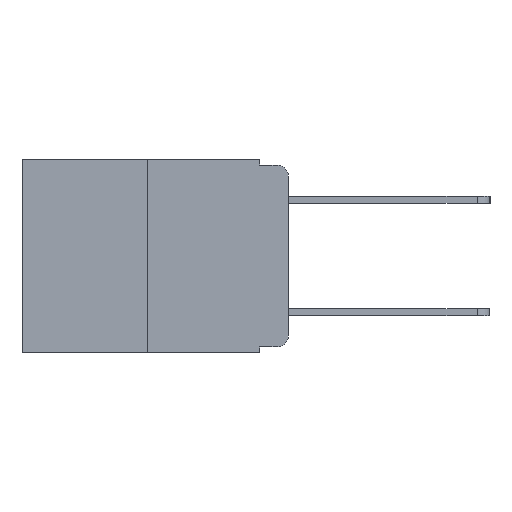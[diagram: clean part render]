
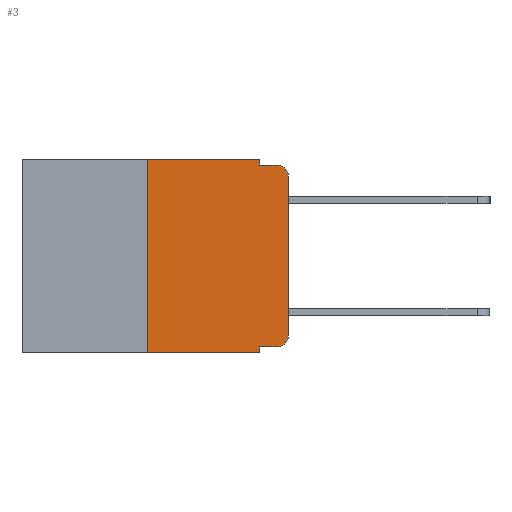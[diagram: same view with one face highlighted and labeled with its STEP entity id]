
A CAD part, left-side view. The second image highlights one B-rep face of the part: STEP entity #3.
In plain terms, the highlighted planar face has unit normal (-1, 0, 0).
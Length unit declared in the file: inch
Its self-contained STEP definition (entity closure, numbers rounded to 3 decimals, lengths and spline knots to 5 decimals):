
#3 = ADVANCED_FACE ( 'NONE', ( #13108 ), #3382, .F. ) ;
#32 = LINE ( 'NONE', #7582, #12911 ) ;
#259 = EDGE_CURVE ( 'NONE', #9305, #6673, #5639, .T. ) ;
#261 = EDGE_CURVE ( 'NONE', #6673, #9650, #8817, .T. ) ;
#316 = EDGE_CURVE ( 'NONE', #12330, #9650, #6974, .T. ) ;
#342 = EDGE_CURVE ( 'NONE', #1228, #12330, #32, .T. ) ;
#355 = AXIS2_PLACEMENT_3D ( 'NONE', #8186, #7905, #7183 ) ;
#370 = EDGE_CURVE ( 'NONE', #1232, #9216, #12588, .T. ) ;
#808 = ORIENTED_EDGE ( 'NONE', *, *, #2164, .F. ) ;
#974 = VERTEX_POINT ( 'NONE', #15124 ) ;
#1061 = CARTESIAN_POINT ( 'NONE',  ( 0., 0.02, -0.313 ) ) ;
#1228 = VERTEX_POINT ( 'NONE', #9665 ) ;
#1232 = VERTEX_POINT ( 'NONE', #15109 ) ;
#1735 = CARTESIAN_POINT ( 'NONE',  ( 0., 0.051, 0. ) ) ;
#2154 = CARTESIAN_POINT ( 'NONE',  ( 0., 0.051, -0.333 ) ) ;
#2164 = EDGE_CURVE ( 'NONE', #9195, #974, #6111, .T. ) ;
#2169 = VECTOR ( 'NONE', #9582, 39.37008 ) ;
#2532 = LINE ( 'NONE', #11211, #11677 ) ;
#2721 = CIRCLE ( 'NONE', #4736, 0.02 ) ;
#2888 = CARTESIAN_POINT ( 'NONE',  ( 0., 0.051, -0.01 ) ) ;
#3136 = AXIS2_PLACEMENT_3D ( 'NONE', #5208, #7556, #10535 ) ;
#3382 = PLANE ( 'NONE',  #3136 ) ;
#3619 = DIRECTION ( 'NONE',  ( -1., 0., 0. ) ) ;
#3633 = VECTOR ( 'NONE', #8522, 39.37008 ) ;
#4021 = EDGE_CURVE ( 'NONE', #9216, #1228, #6920, .T. ) ;
#4278 = EDGE_CURVE ( 'NONE', #9195, #4376, #2532, .T. ) ;
#4324 = CARTESIAN_POINT ( 'NONE',  ( 0., 0.02, -0.333 ) ) ;
#4376 = VERTEX_POINT ( 'NONE', #4324 ) ;
#4663 = EDGE_LOOP ( 'NONE', ( #12659, #4976, #8180, #8531, #5718, #8880, #12145, #808, #5190, #14540 ) ) ;
#4736 = AXIS2_PLACEMENT_3D ( 'NONE', #1061, #3619, #9183 ) ;
#4788 = EDGE_CURVE ( 'NONE', #4376, #9305, #2721, .T. ) ;
#4976 = ORIENTED_EDGE ( 'NONE', *, *, #261, .T. ) ;
#5190 = ORIENTED_EDGE ( 'NONE', *, *, #4278, .T. ) ;
#5208 = CARTESIAN_POINT ( 'NONE',  ( 0., 0.473, 0. ) ) ;
#5300 = CARTESIAN_POINT ( 'NONE',  ( 0., 0.02, -0.01 ) ) ;
#5639 = LINE ( 'NONE', #6180, #2169 ) ;
#5718 = ORIENTED_EDGE ( 'NONE', *, *, #4021, .F. ) ;
#6043 = CARTESIAN_POINT ( 'NONE',  ( 0., 0.25, 0. ) ) ;
#6079 = DIRECTION ( 'NONE',  ( 0., 0., 1. ) ) ;
#6111 = LINE ( 'NONE', #1735, #8557 ) ;
#6117 = CARTESIAN_POINT ( 'NONE',  ( 0., 0.25, 0. ) ) ;
#6153 = CARTESIAN_POINT ( 'NONE',  ( 0., 0., -0.313 ) ) ;
#6180 = CARTESIAN_POINT ( 'NONE',  ( 0., 0., 0. ) ) ;
#6673 = VERTEX_POINT ( 'NONE', #12937 ) ;
#6920 = LINE ( 'NONE', #14701, #12535 ) ;
#6974 = LINE ( 'NONE', #7768, #3633 ) ;
#7183 = DIRECTION ( 'NONE',  ( 0., 0., -1. ) ) ;
#7507 = DIRECTION ( 'NONE',  ( 0., 0., -1. ) ) ;
#7556 = DIRECTION ( 'NONE',  ( 1., 0., 0. ) ) ;
#7582 = CARTESIAN_POINT ( 'NONE',  ( 0., 0.051, 0. ) ) ;
#7768 = CARTESIAN_POINT ( 'NONE',  ( 0., 0.051, -0.01 ) ) ;
#7905 = DIRECTION ( 'NONE',  ( -1., 0., 0. ) ) ;
#8180 = ORIENTED_EDGE ( 'NONE', *, *, #316, .F. ) ;
#8186 = CARTESIAN_POINT ( 'NONE',  ( 0., 0.02, -0.03 ) ) ;
#8205 = DIRECTION ( 'NONE',  ( 0., -1., 0. ) ) ;
#8522 = DIRECTION ( 'NONE',  ( 0., -1., 0. ) ) ;
#8531 = ORIENTED_EDGE ( 'NONE', *, *, #342, .F. ) ;
#8557 = VECTOR ( 'NONE', #14353, 39.37008 ) ;
#8817 = CIRCLE ( 'NONE', #355, 0.02 ) ;
#8880 = ORIENTED_EDGE ( 'NONE', *, *, #370, .F. ) ;
#9183 = DIRECTION ( 'NONE',  ( 0., 0., -1. ) ) ;
#9195 = VERTEX_POINT ( 'NONE', #2154 ) ;
#9216 = VERTEX_POINT ( 'NONE', #6043 ) ;
#9305 = VERTEX_POINT ( 'NONE', #6153 ) ;
#9582 = DIRECTION ( 'NONE',  ( 0., 0., 1. ) ) ;
#9650 = VERTEX_POINT ( 'NONE', #5300 ) ;
#9665 = CARTESIAN_POINT ( 'NONE',  ( 0., 0.051, 0. ) ) ;
#10436 = CARTESIAN_POINT ( 'NONE',  ( 0., 0.473, -0.343 ) ) ;
#10535 = DIRECTION ( 'NONE',  ( 0., 0., -1. ) ) ;
#11211 = CARTESIAN_POINT ( 'NONE',  ( 0., 0.051, -0.333 ) ) ;
#11228 = VECTOR ( 'NONE', #14815, 39.37008 ) ;
#11557 = LINE ( 'NONE', #10436, #11228 ) ;
#11677 = VECTOR ( 'NONE', #8205, 39.37008 ) ;
#12145 = ORIENTED_EDGE ( 'NONE', *, *, #15210, .T. ) ;
#12239 = VECTOR ( 'NONE', #6079, 39.37008 ) ;
#12330 = VERTEX_POINT ( 'NONE', #2888 ) ;
#12535 = VECTOR ( 'NONE', #14593, 39.37008 ) ;
#12588 = LINE ( 'NONE', #6117, #12239 ) ;
#12659 = ORIENTED_EDGE ( 'NONE', *, *, #259, .T. ) ;
#12911 = VECTOR ( 'NONE', #7507, 39.37008 ) ;
#12937 = CARTESIAN_POINT ( 'NONE',  ( 0., 0., -0.03 ) ) ;
#13108 = FACE_OUTER_BOUND ( 'NONE', #4663, .T. ) ;
#14353 = DIRECTION ( 'NONE',  ( 0., 0., -1. ) ) ;
#14540 = ORIENTED_EDGE ( 'NONE', *, *, #4788, .T. ) ;
#14593 = DIRECTION ( 'NONE',  ( 0., -1., 0. ) ) ;
#14701 = CARTESIAN_POINT ( 'NONE',  ( 0., 0.473, 0. ) ) ;
#14815 = DIRECTION ( 'NONE',  ( 0., -1., 0. ) ) ;
#15109 = CARTESIAN_POINT ( 'NONE',  ( 0., 0.25, -0.343 ) ) ;
#15124 = CARTESIAN_POINT ( 'NONE',  ( 0., 0.051, -0.343 ) ) ;
#15210 = EDGE_CURVE ( 'NONE', #1232, #974, #11557, .T. ) ;
